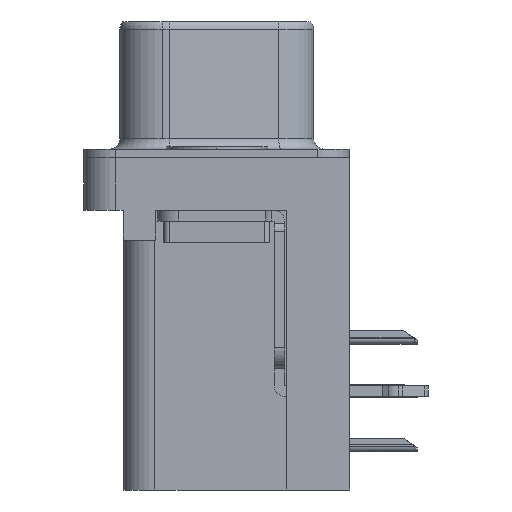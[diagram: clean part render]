
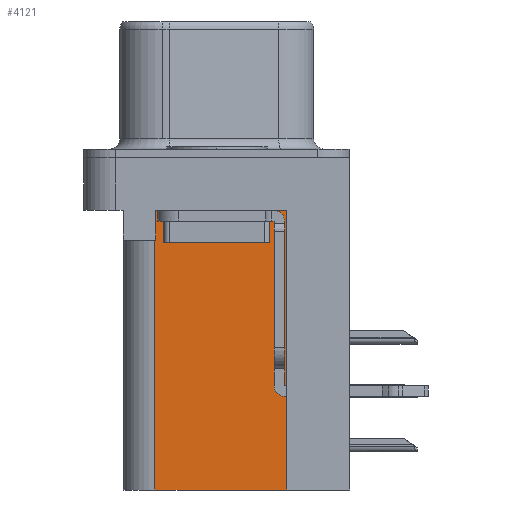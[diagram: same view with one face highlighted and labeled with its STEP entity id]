
A CAD part, left-side view. The second image highlights one B-rep face of the part: STEP entity #4121.
In plain terms, the highlighted planar face has unit normal (-1, 0, 0).
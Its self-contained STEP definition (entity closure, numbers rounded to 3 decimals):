
#331 = ORIENTED_EDGE ( 'NONE', *, *, #355, .T. ) ;
#355 = EDGE_CURVE ( 'NONE', #23021, #24314, #15088, .T. ) ;
#524 = EDGE_CURVE ( 'NONE', #8656, #23021, #23285, .T. ) ;
#1885 = CARTESIAN_POINT ( 'NONE',  ( 3.7, -3.295, -2.5 ) ) ;
#2069 = DIRECTION ( 'NONE',  ( 0., 0., 1. ) ) ;
#2209 = DIRECTION ( 'NONE',  ( 0., 1., 0. ) ) ;
#3678 = VECTOR ( 'NONE', #2209, 1000. ) ;
#3715 = LINE ( 'NONE', #1885, #14454 ) ;
#4121 = ADVANCED_FACE ( 'NONE', ( #10153 ), #5121, .F. ) ;
#4146 = CARTESIAN_POINT ( 'NONE',  ( 3.7, -3.295, -15.7 ) ) ;
#5121 = PLANE ( 'NONE',  #19002 ) ;
#5634 = VECTOR ( 'NONE', #6235, 1000. ) ;
#5898 = ORIENTED_EDGE ( 'NONE', *, *, #10199, .T. ) ;
#6235 = DIRECTION ( 'NONE',  ( 0., 1., 0. ) ) ;
#6416 = CARTESIAN_POINT ( 'NONE',  ( 3.7, 2.895, -3.9 ) ) ;
#6496 = CARTESIAN_POINT ( 'NONE',  ( 3.7, 2.925, -15.7 ) ) ;
#7342 = EDGE_CURVE ( 'NONE', #17875, #8656, #3715, .T. ) ;
#7392 = EDGE_CURVE ( 'NONE', #8568, #24314, #9378, .T. ) ;
#8072 = VECTOR ( 'NONE', #2069, 1000. ) ;
#8505 = CARTESIAN_POINT ( 'NONE',  ( 3.7, 2.895, -3.9 ) ) ;
#8568 = VERTEX_POINT ( 'NONE', #6496 ) ;
#8569 = LINE ( 'NONE', #19655, #20075 ) ;
#8656 = VERTEX_POINT ( 'NONE', #24085 ) ;
#9378 = LINE ( 'NONE', #19199, #8072 ) ;
#10153 = FACE_OUTER_BOUND ( 'NONE', #15824, .T. ) ;
#10199 = EDGE_CURVE ( 'NONE', #23823, #17875, #8569, .T. ) ;
#11007 = VECTOR ( 'NONE', #13895, 1000. ) ;
#13096 = DIRECTION ( 'NONE',  ( 0., 0., 1. ) ) ;
#13361 = CARTESIAN_POINT ( 'NONE',  ( 3.7, 2.925, -3.9 ) ) ;
#13895 = DIRECTION ( 'NONE',  ( 0., 0., -1. ) ) ;
#14454 = VECTOR ( 'NONE', #21343, 1000. ) ;
#15088 = LINE ( 'NONE', #22617, #3678 ) ;
#15824 = EDGE_LOOP ( 'NONE', ( #25157, #19233, #331, #23663, #15930, #5898 ) ) ;
#15930 = ORIENTED_EDGE ( 'NONE', *, *, #24747, .F. ) ;
#17875 = VERTEX_POINT ( 'NONE', #22872 ) ;
#19002 = AXIS2_PLACEMENT_3D ( 'NONE', #4146, #25559, #25597 ) ;
#19199 = CARTESIAN_POINT ( 'NONE',  ( 3.7, 2.925, -15.7 ) ) ;
#19233 = ORIENTED_EDGE ( 'NONE', *, *, #524, .T. ) ;
#19655 = CARTESIAN_POINT ( 'NONE',  ( 3.7, -3.295, -15.7 ) ) ;
#20075 = VECTOR ( 'NONE', #13096, 1000. ) ;
#21343 = DIRECTION ( 'NONE',  ( 0., 1., 0. ) ) ;
#21397 = CARTESIAN_POINT ( 'NONE',  ( 3.7, -3.295, -15.7 ) ) ;
#22617 = CARTESIAN_POINT ( 'NONE',  ( 3.7, 0., -3.9 ) ) ;
#22872 = CARTESIAN_POINT ( 'NONE',  ( 3.7, -3.295, -2.5 ) ) ;
#23021 = VERTEX_POINT ( 'NONE', #8505 ) ;
#23285 = LINE ( 'NONE', #6416, #11007 ) ;
#23663 = ORIENTED_EDGE ( 'NONE', *, *, #7392, .F. ) ;
#23823 = VERTEX_POINT ( 'NONE', #26394 ) ;
#24085 = CARTESIAN_POINT ( 'NONE',  ( 3.7, 2.895, -2.5 ) ) ;
#24314 = VERTEX_POINT ( 'NONE', #13361 ) ;
#24747 = EDGE_CURVE ( 'NONE', #23823, #8568, #27930, .T. ) ;
#25157 = ORIENTED_EDGE ( 'NONE', *, *, #7342, .T. ) ;
#25559 = DIRECTION ( 'NONE',  ( 1., 0., 0. ) ) ;
#25597 = DIRECTION ( 'NONE',  ( 0., 0., -1. ) ) ;
#26394 = CARTESIAN_POINT ( 'NONE',  ( 3.7, -3.295, -15.7 ) ) ;
#27930 = LINE ( 'NONE', #21397, #5634 ) ;
